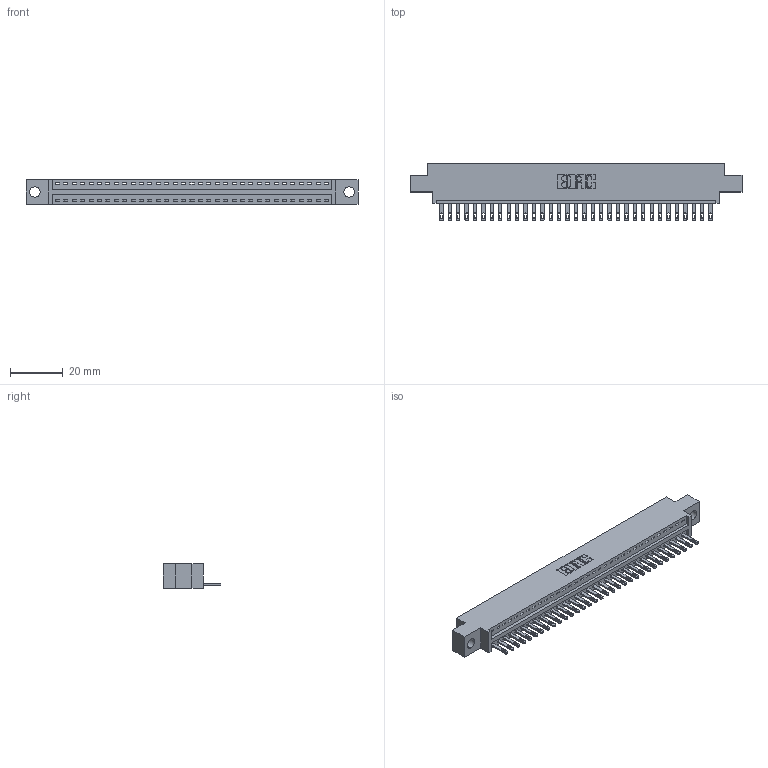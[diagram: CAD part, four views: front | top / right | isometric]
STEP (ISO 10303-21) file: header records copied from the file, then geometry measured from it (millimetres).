
FILE_DESCRIPTION (( 'STEP AP203' ), '1' );
FILE_NAME ('346-033-500-604.STEP', '2022-05-06T19:11:01', ( '' ), ( '' ), 'SwSTEP 2.0', 'SolidWorks 2020', '' );
FILE_SCHEMA (( 'CONFIG_CONTROL_DESIGN' ));
Length unit declared in the file: inch
Products named in the file (3): 346-033-500-604; 346 Part_0.170 Offset - 0.156 Dia-TH; 345-292-001_345-293-100
Assembly tree (34 placements, depth 2):
  346-033-500-604
    346 Part_0.170 Offset - 0.156 Dia-TH
    345-292-001_345-293-100  x33
Bounding box: 125.35 x 21.84 x 9.4 mm (x, y, z)
Volume: 11696.5 mm3; surface area: 14596.5 mm2
Topology: 34 solids, 34 shells, 1922 faces, 5921 edges, 3946 vertices
Faces by surface type: plane 1216, cylinder 706
Entity records: 22173 total; most frequent: CARTESIAN_POINT 3813, ORIENTED_EDGE 3778, DIRECTION 3375, EDGE_CURVE 1889, LINE 1621, VECTOR 1621, VERTEX_POINT 1258, AXIS2_PLACEMENT_3D 877
